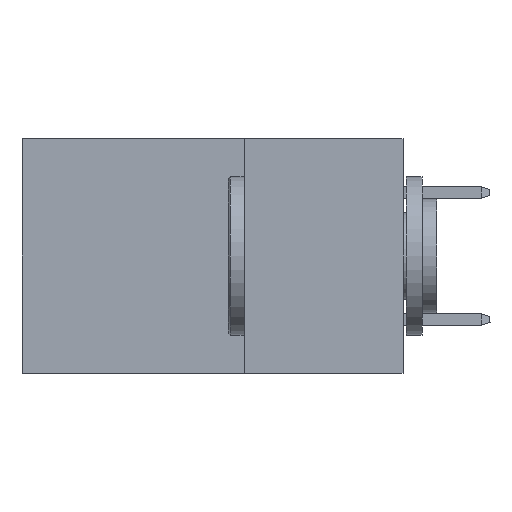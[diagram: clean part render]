
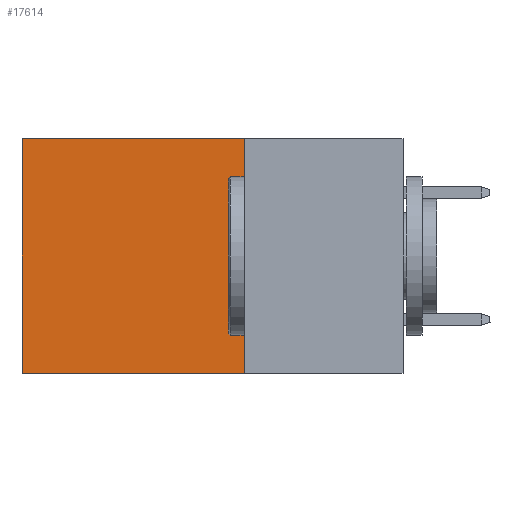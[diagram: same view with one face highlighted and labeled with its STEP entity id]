
A CAD part, left-side view. The second image highlights one B-rep face of the part: STEP entity #17614.
In plain terms, the highlighted planar face has unit normal (-1, 0, 0).
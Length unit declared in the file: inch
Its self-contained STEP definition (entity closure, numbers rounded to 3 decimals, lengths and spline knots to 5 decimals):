
#440 = DIRECTION ( 'NONE',  ( 0., 0., -1. ) ) ;
#1042 = AXIS2_PLACEMENT_3D ( 'NONE', #15282, #5448, #11057 ) ;
#1207 = DIRECTION ( 'NONE',  ( 0., 0., -1. ) ) ;
#1783 = ORIENTED_EDGE ( 'NONE', *, *, #5970, .T. ) ;
#2391 = CARTESIAN_POINT ( 'NONE',  ( 0.2875, 0.6, 0. ) ) ;
#2694 = DIRECTION ( 'NONE',  ( 0., 1., 0. ) ) ;
#4104 = ORIENTED_EDGE ( 'NONE', *, *, #13803, .T. ) ;
#4798 = EDGE_CURVE ( 'NONE', #8399, #8149, #14329, .T. ) ;
#5448 = DIRECTION ( 'NONE',  ( 1., 0., 0. ) ) ;
#5691 = VERTEX_POINT ( 'NONE', #7468 ) ;
#5701 = DIRECTION ( 'NONE',  ( 0., 1., 0. ) ) ;
#5970 = EDGE_CURVE ( 'NONE', #8399, #9238, #12693, .T. ) ;
#6313 = CARTESIAN_POINT ( 'NONE',  ( 0.2875, 0.25, 0. ) ) ;
#6823 = LINE ( 'NONE', #9790, #15412 ) ;
#7022 = FACE_OUTER_BOUND ( 'NONE', #14178, .T. ) ;
#7347 = CARTESIAN_POINT ( 'NONE',  ( 0.2875, 0.25, 0. ) ) ;
#7468 = CARTESIAN_POINT ( 'NONE',  ( 0.2875, 0.6, -0.37 ) ) ;
#8149 = VERTEX_POINT ( 'NONE', #15322 ) ;
#8178 = VECTOR ( 'NONE', #440, 39.37008 ) ;
#8399 = VERTEX_POINT ( 'NONE', #6313 ) ;
#8490 = CARTESIAN_POINT ( 'NONE',  ( 0.2875, 0.25, 0. ) ) ;
#9080 = VECTOR ( 'NONE', #1207, 39.37008 ) ;
#9126 = VECTOR ( 'NONE', #5701, 39.37008 ) ;
#9238 = VERTEX_POINT ( 'NONE', #2391 ) ;
#9790 = CARTESIAN_POINT ( 'NONE',  ( 0.2875, 0.25, -0.37 ) ) ;
#10613 = LINE ( 'NONE', #16359, #9080 ) ;
#10742 = EDGE_CURVE ( 'NONE', #8149, #5691, #6823, .T. ) ;
#10821 = ORIENTED_EDGE ( 'NONE', *, *, #10742, .F. ) ;
#11057 = DIRECTION ( 'NONE',  ( 0., 0., -1. ) ) ;
#12693 = LINE ( 'NONE', #8490, #9126 ) ;
#13803 = EDGE_CURVE ( 'NONE', #9238, #5691, #10613, .T. ) ;
#14178 = EDGE_LOOP ( 'NONE', ( #4104, #10821, #15956, #1783 ) ) ;
#14329 = LINE ( 'NONE', #7347, #8178 ) ;
#15282 = CARTESIAN_POINT ( 'NONE',  ( 0.2875, 0.25, 0. ) ) ;
#15322 = CARTESIAN_POINT ( 'NONE',  ( 0.2875, 0.25, -0.37 ) ) ;
#15412 = VECTOR ( 'NONE', #2694, 39.37008 ) ;
#15956 = ORIENTED_EDGE ( 'NONE', *, *, #4798, .F. ) ;
#16359 = CARTESIAN_POINT ( 'NONE',  ( 0.2875, 0.6, 0. ) ) ;
#17614 = ADVANCED_FACE ( 'NONE', ( #7022 ), #17997, .F. ) ;
#17997 = PLANE ( 'NONE',  #1042 ) ;
